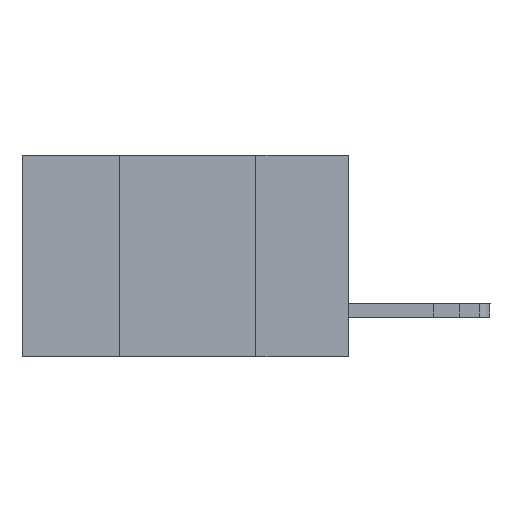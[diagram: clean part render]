
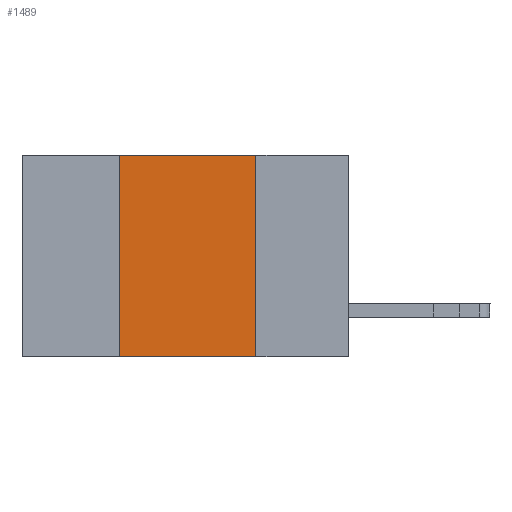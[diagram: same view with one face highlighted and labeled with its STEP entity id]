
A CAD part, left-side view. The second image highlights one B-rep face of the part: STEP entity #1489.
In plain terms, the highlighted planar face has unit normal (-1, 0, 0).
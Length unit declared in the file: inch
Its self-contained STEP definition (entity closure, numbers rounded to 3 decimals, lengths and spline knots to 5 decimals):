
#168 = VECTOR ( 'NONE', #10673, 39.37008 ) ;
#361 = VERTEX_POINT ( 'NONE', #9192 ) ;
#465 = EDGE_LOOP ( 'NONE', ( #7581, #2435, #5629, #9375 ) ) ;
#658 = DIRECTION ( 'NONE',  ( 0., 0., -1. ) ) ;
#1468 = PLANE ( 'NONE',  #12316 ) ;
#1489 = ADVANCED_FACE ( 'NONE', ( #4520 ), #1468, .F. ) ;
#1506 = VECTOR ( 'NONE', #4074, 39.37008 ) ;
#1857 = VECTOR ( 'NONE', #11571, 39.37008 ) ;
#2009 = CARTESIAN_POINT ( 'NONE',  ( 0., 0.17, -0.37 ) ) ;
#2029 = VERTEX_POINT ( 'NONE', #9687 ) ;
#2435 = ORIENTED_EDGE ( 'NONE', *, *, #4763, .F. ) ;
#3453 = CARTESIAN_POINT ( 'NONE',  ( 0., 0.42, -0.37 ) ) ;
#4074 = DIRECTION ( 'NONE',  ( 0., 0., 1. ) ) ;
#4246 = DIRECTION ( 'NONE',  ( 1., 0., 0. ) ) ;
#4506 = CARTESIAN_POINT ( 'NONE',  ( 0., 0.17, -0.37 ) ) ;
#4520 = FACE_OUTER_BOUND ( 'NONE', #465, .T. ) ;
#4763 = EDGE_CURVE ( 'NONE', #361, #2029, #10082, .T. ) ;
#5196 = EDGE_CURVE ( 'NONE', #10910, #361, #9747, .T. ) ;
#5607 = DIRECTION ( 'NONE',  ( 0., -1., 0. ) ) ;
#5629 = ORIENTED_EDGE ( 'NONE', *, *, #5196, .F. ) ;
#7581 = ORIENTED_EDGE ( 'NONE', *, *, #9352, .F. ) ;
#7641 = CARTESIAN_POINT ( 'NONE',  ( 0., 0.6, -0.37 ) ) ;
#8470 = CARTESIAN_POINT ( 'NONE',  ( 0., 0.42, -0.37 ) ) ;
#9192 = CARTESIAN_POINT ( 'NONE',  ( 0., 0.42, 0. ) ) ;
#9352 = EDGE_CURVE ( 'NONE', #2029, #12317, #10758, .T. ) ;
#9375 = ORIENTED_EDGE ( 'NONE', *, *, #9887, .T. ) ;
#9687 = CARTESIAN_POINT ( 'NONE',  ( 0., 0.17, 0. ) ) ;
#9747 = LINE ( 'NONE', #3453, #1506 ) ;
#9803 = LINE ( 'NONE', #7641, #12148 ) ;
#9887 = EDGE_CURVE ( 'NONE', #10910, #12317, #9803, .T. ) ;
#10082 = LINE ( 'NONE', #11901, #1857 ) ;
#10673 = DIRECTION ( 'NONE',  ( 0., 0., -1. ) ) ;
#10758 = LINE ( 'NONE', #4506, #168 ) ;
#10910 = VERTEX_POINT ( 'NONE', #8470 ) ;
#11513 = CARTESIAN_POINT ( 'NONE',  ( 0., 0.6, 0. ) ) ;
#11571 = DIRECTION ( 'NONE',  ( 0., -1., 0. ) ) ;
#11901 = CARTESIAN_POINT ( 'NONE',  ( 0., 0.6, 0. ) ) ;
#12148 = VECTOR ( 'NONE', #5607, 39.37008 ) ;
#12316 = AXIS2_PLACEMENT_3D ( 'NONE', #11513, #4246, #658 ) ;
#12317 = VERTEX_POINT ( 'NONE', #2009 ) ;
